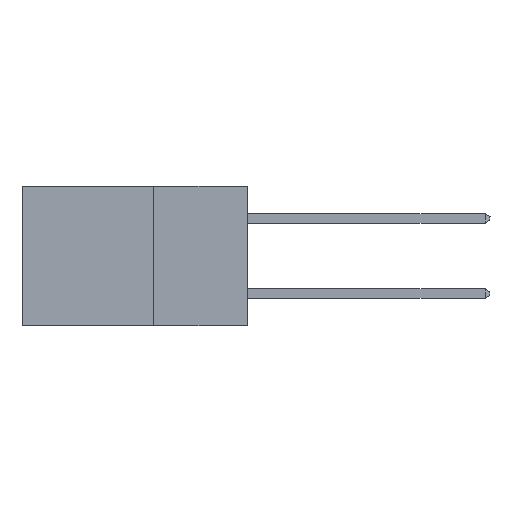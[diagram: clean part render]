
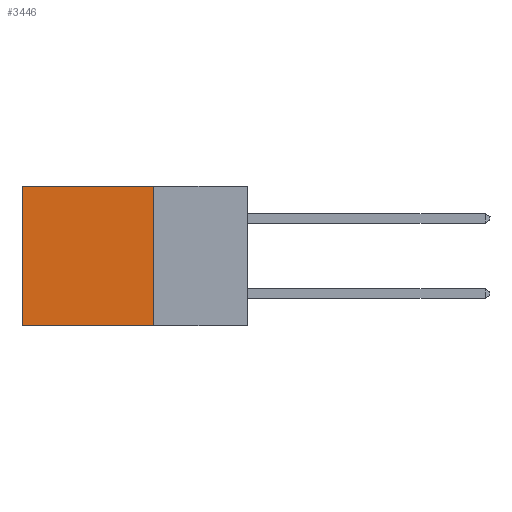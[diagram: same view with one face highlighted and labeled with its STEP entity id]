
A CAD part, left-side view. The second image highlights one B-rep face of the part: STEP entity #3446.
In plain terms, the highlighted planar face has unit normal (-1, 0, 0).
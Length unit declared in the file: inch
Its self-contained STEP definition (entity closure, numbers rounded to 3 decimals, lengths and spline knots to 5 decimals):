
#66 = CARTESIAN_POINT ( 'NONE',  ( 0.2615, 0.6, 0. ) ) ;
#182 = VERTEX_POINT ( 'NONE', #66 ) ;
#339 = CARTESIAN_POINT ( 'NONE',  ( 0.2615, 0.25, -0.37 ) ) ;
#1964 = ORIENTED_EDGE ( 'NONE', *, *, #4673, .F. ) ;
#2098 = ORIENTED_EDGE ( 'NONE', *, *, #6670, .F. ) ;
#3446 = ADVANCED_FACE ( 'NONE', ( #17254 ), #9358, .F. ) ;
#3518 = EDGE_CURVE ( 'NONE', #8285, #182, #6711, .T. ) ;
#4257 = LINE ( 'NONE', #10069, #8505 ) ;
#4469 = CARTESIAN_POINT ( 'NONE',  ( 0.2615, 0.6, -0.37 ) ) ;
#4673 = EDGE_CURVE ( 'NONE', #8285, #7369, #13602, .T. ) ;
#5569 = DIRECTION ( 'NONE',  ( 0., 1., 0. ) ) ;
#6099 = DIRECTION ( 'NONE',  ( 0., 0., -1. ) ) ;
#6670 = EDGE_CURVE ( 'NONE', #7369, #16559, #10233, .T. ) ;
#6711 = LINE ( 'NONE', #12881, #15550 ) ;
#7369 = VERTEX_POINT ( 'NONE', #339 ) ;
#7727 = DIRECTION ( 'NONE',  ( 1., 0., 0. ) ) ;
#8285 = VERTEX_POINT ( 'NONE', #16734 ) ;
#8505 = VECTOR ( 'NONE', #16536, 39.37008 ) ;
#9358 = PLANE ( 'NONE',  #14571 ) ;
#10069 = CARTESIAN_POINT ( 'NONE',  ( 0.2615, 0.6, -0.37 ) ) ;
#10233 = LINE ( 'NONE', #19441, #19120 ) ;
#10272 = DIRECTION ( 'NONE',  ( 0., 0., -1. ) ) ;
#10363 = EDGE_CURVE ( 'NONE', #182, #16559, #4257, .T. ) ;
#11507 = ORIENTED_EDGE ( 'NONE', *, *, #3518, .T. ) ;
#12501 = ORIENTED_EDGE ( 'NONE', *, *, #10363, .T. ) ;
#12576 = EDGE_LOOP ( 'NONE', ( #12501, #2098, #1964, #11507 ) ) ;
#12881 = CARTESIAN_POINT ( 'NONE',  ( 0.2615, 0.25, 0. ) ) ;
#13171 = DIRECTION ( 'NONE',  ( 0., 1., 0. ) ) ;
#13602 = LINE ( 'NONE', #19684, #16822 ) ;
#14571 = AXIS2_PLACEMENT_3D ( 'NONE', #15426, #7727, #6099 ) ;
#15426 = CARTESIAN_POINT ( 'NONE',  ( 0.2615, 0.25, -0.37 ) ) ;
#15550 = VECTOR ( 'NONE', #13171, 39.37008 ) ;
#16536 = DIRECTION ( 'NONE',  ( 0., 0., -1. ) ) ;
#16559 = VERTEX_POINT ( 'NONE', #4469 ) ;
#16734 = CARTESIAN_POINT ( 'NONE',  ( 0.2615, 0.25, 0. ) ) ;
#16822 = VECTOR ( 'NONE', #10272, 39.37008 ) ;
#17254 = FACE_OUTER_BOUND ( 'NONE', #12576, .T. ) ;
#19120 = VECTOR ( 'NONE', #5569, 39.37008 ) ;
#19441 = CARTESIAN_POINT ( 'NONE',  ( 0.2615, 0.25, -0.37 ) ) ;
#19684 = CARTESIAN_POINT ( 'NONE',  ( 0.2615, 0.25, -0.37 ) ) ;
